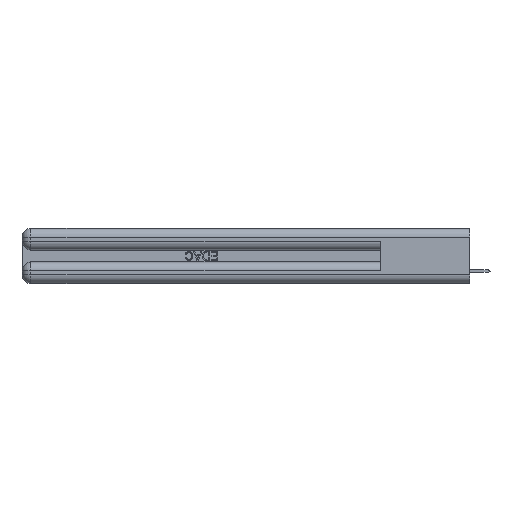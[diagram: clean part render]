
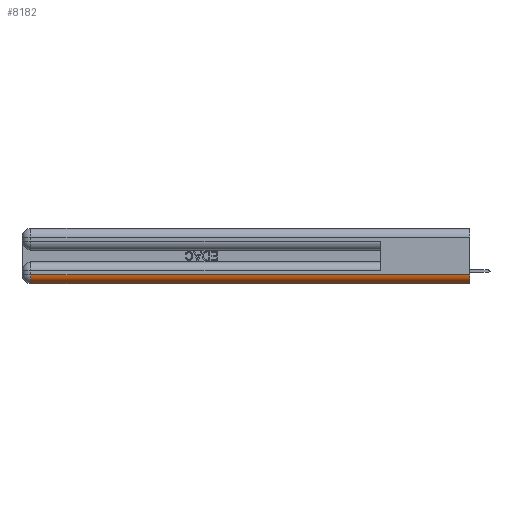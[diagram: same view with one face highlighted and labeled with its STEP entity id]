
A CAD part, left-side view. The second image highlights one B-rep face of the part: STEP entity #8182.
In plain terms, the highlighted cylindrical face has radius 1.524 mm (diameter 3.048 mm), a partial arc.
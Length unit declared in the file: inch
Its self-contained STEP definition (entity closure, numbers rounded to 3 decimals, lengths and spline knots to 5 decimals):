
#1765 = VERTEX_POINT ( 'NONE', #27474 ) ;
#2550 = DIRECTION ( 'NONE',  ( 0., 1., 0. ) ) ;
#2751 = CARTESIAN_POINT ( 'NONE',  ( 0.06, 2.94, 0.06 ) ) ;
#2828 = ORIENTED_EDGE ( 'NONE', *, *, #31771, .F. ) ;
#5108 = VECTOR ( 'NONE', #5299, 39.37008 ) ;
#5299 = DIRECTION ( 'NONE',  ( 0., -1., 0. ) ) ;
#5533 = VERTEX_POINT ( 'NONE', #22390 ) ;
#7152 = AXIS2_PLACEMENT_3D ( 'NONE', #34194, #21665, #36730 ) ;
#8182 = ADVANCED_FACE ( 'NONE', ( #20960 ), #33464, .T. ) ;
#8339 = EDGE_CURVE ( 'NONE', #11921, #5533, #34070, .T. ) ;
#8403 = AXIS2_PLACEMENT_3D ( 'NONE', #33033, #32828, #16991 ) ;
#11545 = LINE ( 'NONE', #24248, #15657 ) ;
#11877 = EDGE_CURVE ( 'NONE', #1765, #18015, #11545, .T. ) ;
#11921 = VERTEX_POINT ( 'NONE', #21912 ) ;
#14529 = ORIENTED_EDGE ( 'NONE', *, *, #11877, .F. ) ;
#15657 = VECTOR ( 'NONE', #36993, 39.37008 ) ;
#16991 = DIRECTION ( 'NONE',  ( 0., 0., 1. ) ) ;
#18015 = VERTEX_POINT ( 'NONE', #24017 ) ;
#19822 = CIRCLE ( 'NONE', #7152, 0.06 ) ;
#20847 = ORIENTED_EDGE ( 'NONE', *, *, #31008, .F. ) ;
#20960 = FACE_OUTER_BOUND ( 'NONE', #39573, .T. ) ;
#21665 = DIRECTION ( 'NONE',  ( 0., -1., 0. ) ) ;
#21714 = DIRECTION ( 'NONE',  ( 0., 0., 1. ) ) ;
#21912 = CARTESIAN_POINT ( 'NONE',  ( 0., 2.94, 0.06 ) ) ;
#22390 = CARTESIAN_POINT ( 'NONE',  ( 0., 0., 0.06 ) ) ;
#24017 = CARTESIAN_POINT ( 'NONE',  ( 0.06, 2.94, 0. ) ) ;
#24248 = CARTESIAN_POINT ( 'NONE',  ( 0.06, 3., 0. ) ) ;
#26485 = ORIENTED_EDGE ( 'NONE', *, *, #8339, .F. ) ;
#27474 = CARTESIAN_POINT ( 'NONE',  ( 0.06, 0., 0. ) ) ;
#30547 = AXIS2_PLACEMENT_3D ( 'NONE', #2751, #2550, #21714 ) ;
#31008 = EDGE_CURVE ( 'NONE', #5533, #1765, #19822, .T. ) ;
#31771 = EDGE_CURVE ( 'NONE', #18015, #11921, #37851, .T. ) ;
#32828 = DIRECTION ( 'NONE',  ( 0., 1., 0. ) ) ;
#33033 = CARTESIAN_POINT ( 'NONE',  ( 0.06, 0., 0.06 ) ) ;
#33464 = CYLINDRICAL_SURFACE ( 'NONE', #8403, 0.06 ) ;
#34070 = LINE ( 'NONE', #34275, #5108 ) ;
#34194 = CARTESIAN_POINT ( 'NONE',  ( 0.06, 0., 0.06 ) ) ;
#34275 = CARTESIAN_POINT ( 'NONE',  ( 0., 0., 0.06 ) ) ;
#36730 = DIRECTION ( 'NONE',  ( 0., 0., 1. ) ) ;
#36993 = DIRECTION ( 'NONE',  ( 0., 1., 0. ) ) ;
#37851 = CIRCLE ( 'NONE', #30547, 0.06 ) ;
#39573 = EDGE_LOOP ( 'NONE', ( #20847, #26485, #2828, #14529 ) ) ;
